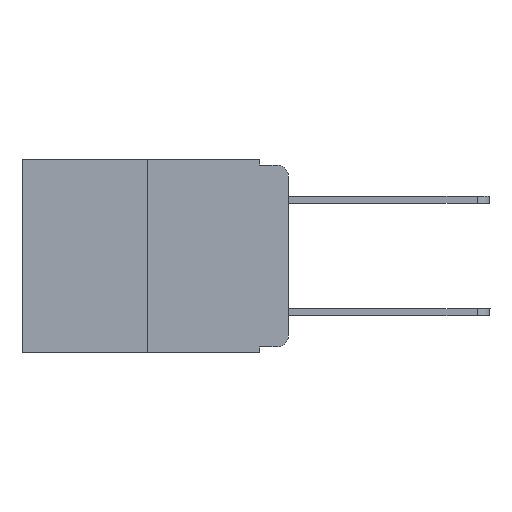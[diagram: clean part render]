
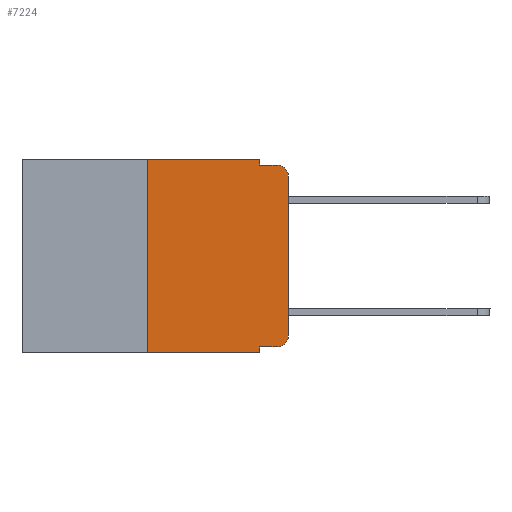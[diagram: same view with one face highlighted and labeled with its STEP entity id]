
A CAD part, left-side view. The second image highlights one B-rep face of the part: STEP entity #7224.
In plain terms, the highlighted planar face has unit normal (-1, 0, 0).
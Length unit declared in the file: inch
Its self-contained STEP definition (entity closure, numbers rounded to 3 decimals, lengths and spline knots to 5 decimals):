
#175 = CARTESIAN_POINT ( 'NONE',  ( 0., 0.25, 0. ) ) ;
#229 = VERTEX_POINT ( 'NONE', #737 ) ;
#418 = CARTESIAN_POINT ( 'NONE',  ( 0., 0.473, 0. ) ) ;
#467 = PLANE ( 'NONE',  #10627 ) ;
#737 = CARTESIAN_POINT ( 'NONE',  ( 0., 0.051, -0.343 ) ) ;
#1006 = ORIENTED_EDGE ( 'NONE', *, *, #1189, .T. ) ;
#1086 = LINE ( 'NONE', #8709, #9858 ) ;
#1147 = VERTEX_POINT ( 'NONE', #12765 ) ;
#1189 = EDGE_CURVE ( 'NONE', #14387, #4894, #6619, .T. ) ;
#1843 = VERTEX_POINT ( 'NONE', #10717 ) ;
#1850 = LINE ( 'NONE', #6378, #11135 ) ;
#2049 = DIRECTION ( 'NONE',  ( -1., 0., 0. ) ) ;
#2056 = EDGE_CURVE ( 'NONE', #10328, #229, #4460, .T. ) ;
#2141 = VERTEX_POINT ( 'NONE', #4648 ) ;
#2305 = EDGE_LOOP ( 'NONE', ( #1006, #11292, #2777, #5754, #9259, #8780, #7340, #12039, #9723, #2466 ) ) ;
#2429 = CARTESIAN_POINT ( 'NONE',  ( 0., 0., -0.313 ) ) ;
#2466 = ORIENTED_EDGE ( 'NONE', *, *, #8811, .T. ) ;
#2526 = EDGE_CURVE ( 'NONE', #4894, #2141, #12824, .T. ) ;
#2622 = EDGE_CURVE ( 'NONE', #10328, #1147, #5844, .T. ) ;
#2777 = ORIENTED_EDGE ( 'NONE', *, *, #8834, .F. ) ;
#3339 = EDGE_CURVE ( 'NONE', #1843, #13633, #11018, .T. ) ;
#3949 = DIRECTION ( 'NONE',  ( 0., 0., 1. ) ) ;
#4351 = CIRCLE ( 'NONE', #13863, 0.02 ) ;
#4377 = CARTESIAN_POINT ( 'NONE',  ( 0., 0.051, -0.01 ) ) ;
#4460 = LINE ( 'NONE', #5345, #11056 ) ;
#4648 = CARTESIAN_POINT ( 'NONE',  ( 0., 0.02, -0.01 ) ) ;
#4894 = VERTEX_POINT ( 'NONE', #8388 ) ;
#5080 = EDGE_CURVE ( 'NONE', #10701, #11648, #6237, .T. ) ;
#5345 = CARTESIAN_POINT ( 'NONE',  ( 0., 0.051, 0. ) ) ;
#5754 = ORIENTED_EDGE ( 'NONE', *, *, #5080, .F. ) ;
#5803 = CARTESIAN_POINT ( 'NONE',  ( 0., 0., 0. ) ) ;
#5844 = LINE ( 'NONE', #11416, #10695 ) ;
#6237 = LINE ( 'NONE', #7365, #7155 ) ;
#6276 = VECTOR ( 'NONE', #12993, 39.37008 ) ;
#6378 = CARTESIAN_POINT ( 'NONE',  ( 0., 0.051, -0.01 ) ) ;
#6619 = LINE ( 'NONE', #5803, #10199 ) ;
#7155 = VECTOR ( 'NONE', #10962, 39.37008 ) ;
#7224 = ADVANCED_FACE ( 'NONE', ( #8415 ), #467, .F. ) ;
#7340 = ORIENTED_EDGE ( 'NONE', *, *, #10444, .T. ) ;
#7365 = CARTESIAN_POINT ( 'NONE',  ( 0., 0.051, 0. ) ) ;
#7537 = AXIS2_PLACEMENT_3D ( 'NONE', #9769, #11515, #12325 ) ;
#7667 = DIRECTION ( 'NONE',  ( 0., 0., -1. ) ) ;
#8182 = VECTOR ( 'NONE', #3949, 39.37008 ) ;
#8184 = DIRECTION ( 'NONE',  ( 1., 0., 0. ) ) ;
#8388 = CARTESIAN_POINT ( 'NONE',  ( 0., 0., -0.03 ) ) ;
#8415 = FACE_OUTER_BOUND ( 'NONE', #2305, .T. ) ;
#8709 = CARTESIAN_POINT ( 'NONE',  ( 0., 0.473, -0.343 ) ) ;
#8758 = DIRECTION ( 'NONE',  ( 0., -1., 0. ) ) ;
#8780 = ORIENTED_EDGE ( 'NONE', *, *, #3339, .F. ) ;
#8811 = EDGE_CURVE ( 'NONE', #1147, #14387, #4351, .T. ) ;
#8834 = EDGE_CURVE ( 'NONE', #11648, #2141, #1850, .T. ) ;
#9259 = ORIENTED_EDGE ( 'NONE', *, *, #9707, .F. ) ;
#9707 = EDGE_CURVE ( 'NONE', #13633, #10701, #13251, .T. ) ;
#9723 = ORIENTED_EDGE ( 'NONE', *, *, #2622, .T. ) ;
#9769 = CARTESIAN_POINT ( 'NONE',  ( 0., 0.02, -0.03 ) ) ;
#9833 = DIRECTION ( 'NONE',  ( 0., -1., 0. ) ) ;
#9858 = VECTOR ( 'NONE', #8758, 39.37008 ) ;
#10199 = VECTOR ( 'NONE', #12955, 39.37008 ) ;
#10328 = VERTEX_POINT ( 'NONE', #14132 ) ;
#10444 = EDGE_CURVE ( 'NONE', #1843, #229, #1086, .T. ) ;
#10627 = AXIS2_PLACEMENT_3D ( 'NONE', #12702, #8184, #7667 ) ;
#10695 = VECTOR ( 'NONE', #12662, 39.37008 ) ;
#10701 = VERTEX_POINT ( 'NONE', #13818 ) ;
#10717 = CARTESIAN_POINT ( 'NONE',  ( 0., 0.25, -0.343 ) ) ;
#10962 = DIRECTION ( 'NONE',  ( 0., 0., -1. ) ) ;
#11018 = LINE ( 'NONE', #13008, #8182 ) ;
#11056 = VECTOR ( 'NONE', #11144, 39.37008 ) ;
#11135 = VECTOR ( 'NONE', #9833, 39.37008 ) ;
#11144 = DIRECTION ( 'NONE',  ( 0., 0., -1. ) ) ;
#11175 = DIRECTION ( 'NONE',  ( 0., 0., -1. ) ) ;
#11292 = ORIENTED_EDGE ( 'NONE', *, *, #2526, .T. ) ;
#11416 = CARTESIAN_POINT ( 'NONE',  ( 0., 0.051, -0.333 ) ) ;
#11515 = DIRECTION ( 'NONE',  ( -1., 0., 0. ) ) ;
#11648 = VERTEX_POINT ( 'NONE', #4377 ) ;
#12039 = ORIENTED_EDGE ( 'NONE', *, *, #2056, .F. ) ;
#12325 = DIRECTION ( 'NONE',  ( 0., 0., -1. ) ) ;
#12662 = DIRECTION ( 'NONE',  ( 0., -1., 0. ) ) ;
#12702 = CARTESIAN_POINT ( 'NONE',  ( 0., 0.473, 0. ) ) ;
#12765 = CARTESIAN_POINT ( 'NONE',  ( 0., 0.02, -0.333 ) ) ;
#12824 = CIRCLE ( 'NONE', #7537, 0.02 ) ;
#12955 = DIRECTION ( 'NONE',  ( 0., 0., 1. ) ) ;
#12993 = DIRECTION ( 'NONE',  ( 0., -1., 0. ) ) ;
#13008 = CARTESIAN_POINT ( 'NONE',  ( 0., 0.25, 0. ) ) ;
#13251 = LINE ( 'NONE', #418, #6276 ) ;
#13426 = CARTESIAN_POINT ( 'NONE',  ( 0., 0.02, -0.313 ) ) ;
#13633 = VERTEX_POINT ( 'NONE', #175 ) ;
#13818 = CARTESIAN_POINT ( 'NONE',  ( 0., 0.051, 0. ) ) ;
#13863 = AXIS2_PLACEMENT_3D ( 'NONE', #13426, #2049, #11175 ) ;
#14132 = CARTESIAN_POINT ( 'NONE',  ( 0., 0.051, -0.333 ) ) ;
#14387 = VERTEX_POINT ( 'NONE', #2429 ) ;
